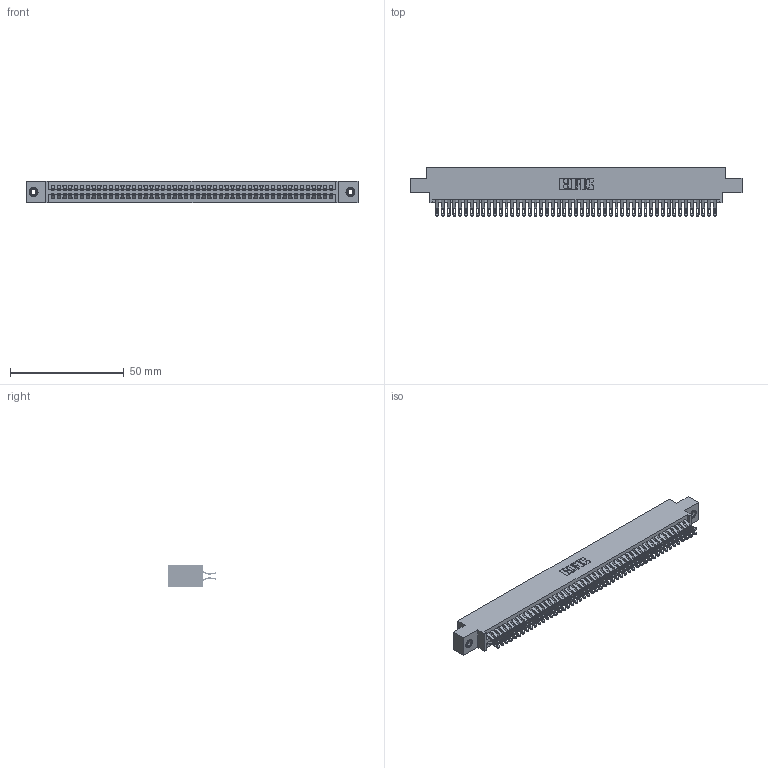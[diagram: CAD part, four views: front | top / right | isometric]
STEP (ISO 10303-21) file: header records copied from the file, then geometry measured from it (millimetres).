
FILE_DESCRIPTION (( 'STEP AP203' ), '1' );
FILE_NAME ('395-098-555-808.STEP', '2018-11-29T21:49:02', ( '' ), ( '' ), 'SwSTEP 2.0', 'SolidWorks 2016', '' );
FILE_SCHEMA (( 'CONFIG_CONTROL_DESIGN' ));
Length unit declared in the file: inch
Products named in the file (4): 395-098-555-808; 345 Part_0.170 Offset - 0.156 Dia-TI; 345-250-001_345-250-003-102; 345-292-001_555 Tail
Assembly tree (101 placements, depth 2):
  395-098-555-808
    345 Part_0.170 Offset - 0.156 Dia-TI
    345-292-001_555 Tail  x98
    345-250-001_345-250-003-102  x2
Bounding box: 145.67 x 21.13 x 9.4 mm (x, y, z)
Volume: 14379.8 mm3; surface area: 22536.8 mm2
Topology: 101 solids, 101 shells, 5678 faces, 17835 edges, 11882 vertices
Faces by surface type: plane 3154, cylinder 2508, cone 12, torus 4
Entity records: 39148 total; most frequent: CARTESIAN_POINT 6573, ORIENTED_EDGE 6470, DIRECTION 5781, EDGE_CURVE 3235, LINE 2867, VECTOR 2867, VERTEX_POINT 2152, AXIS2_PLACEMENT_3D 1457
